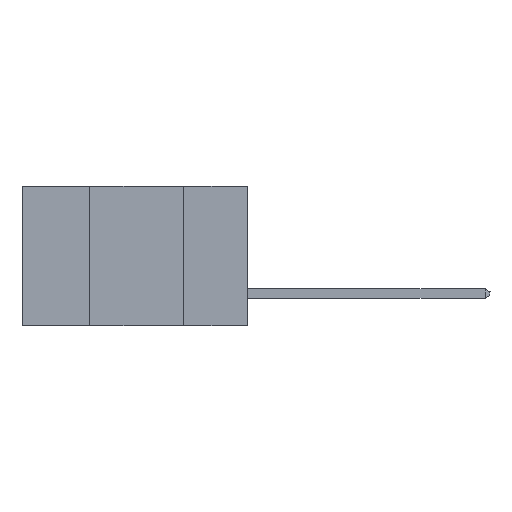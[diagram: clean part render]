
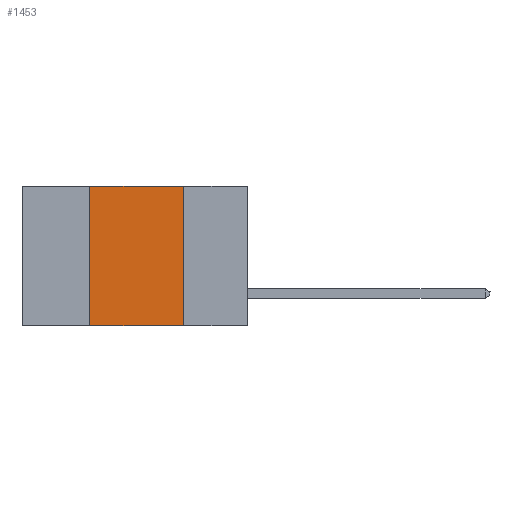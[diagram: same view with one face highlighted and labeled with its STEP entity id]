
A CAD part, left-side view. The second image highlights one B-rep face of the part: STEP entity #1453.
In plain terms, the highlighted planar face has unit normal (-1, 0, 0).
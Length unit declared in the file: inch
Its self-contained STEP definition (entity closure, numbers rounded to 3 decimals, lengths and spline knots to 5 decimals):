
#196 = DIRECTION ( 'NONE',  ( 0., -1., 0. ) ) ;
#423 = LINE ( 'NONE', #4731, #7227 ) ;
#1056 = VECTOR ( 'NONE', #19698, 39.37008 ) ;
#1349 = VERTEX_POINT ( 'NONE', #10973 ) ;
#1453 = ADVANCED_FACE ( 'NONE', ( #17598 ), #8153, .F. ) ;
#1739 = DIRECTION ( 'NONE',  ( 0., -1., 0. ) ) ;
#3515 = DIRECTION ( 'NONE',  ( 0., 0., -1. ) ) ;
#4006 = VERTEX_POINT ( 'NONE', #19813 ) ;
#4731 = CARTESIAN_POINT ( 'NONE',  ( 0., 0.17, -0.37 ) ) ;
#5026 = CARTESIAN_POINT ( 'NONE',  ( 0., 0.6, 0. ) ) ;
#5100 = LINE ( 'NONE', #5406, #1056 ) ;
#5406 = CARTESIAN_POINT ( 'NONE',  ( 0., 0.42, -0.37 ) ) ;
#6451 = CARTESIAN_POINT ( 'NONE',  ( 0., 0.6, 0. ) ) ;
#7102 = CARTESIAN_POINT ( 'NONE',  ( 0., 0.17, -0.37 ) ) ;
#7209 = EDGE_LOOP ( 'NONE', ( #10564, #15034, #8240, #12694 ) ) ;
#7227 = VECTOR ( 'NONE', #11128, 39.37008 ) ;
#7438 = VECTOR ( 'NONE', #196, 39.37008 ) ;
#8153 = PLANE ( 'NONE',  #9838 ) ;
#8240 = ORIENTED_EDGE ( 'NONE', *, *, #19629, .F. ) ;
#8712 = LINE ( 'NONE', #5026, #7438 ) ;
#9267 = EDGE_CURVE ( 'NONE', #4006, #17604, #423, .T. ) ;
#9838 = AXIS2_PLACEMENT_3D ( 'NONE', #6451, #9941, #3515 ) ;
#9941 = DIRECTION ( 'NONE',  ( 1., 0., 0. ) ) ;
#10063 = LINE ( 'NONE', #10166, #12621 ) ;
#10166 = CARTESIAN_POINT ( 'NONE',  ( 0., 0.6, -0.37 ) ) ;
#10564 = ORIENTED_EDGE ( 'NONE', *, *, #9267, .F. ) ;
#10910 = EDGE_CURVE ( 'NONE', #1349, #17604, #10063, .T. ) ;
#10973 = CARTESIAN_POINT ( 'NONE',  ( 0., 0.42, -0.37 ) ) ;
#11043 = VERTEX_POINT ( 'NONE', #13222 ) ;
#11128 = DIRECTION ( 'NONE',  ( 0., 0., -1. ) ) ;
#12621 = VECTOR ( 'NONE', #1739, 39.37008 ) ;
#12694 = ORIENTED_EDGE ( 'NONE', *, *, #10910, .T. ) ;
#13222 = CARTESIAN_POINT ( 'NONE',  ( 0., 0.42, 0. ) ) ;
#15034 = ORIENTED_EDGE ( 'NONE', *, *, #17180, .F. ) ;
#17180 = EDGE_CURVE ( 'NONE', #11043, #4006, #8712, .T. ) ;
#17598 = FACE_OUTER_BOUND ( 'NONE', #7209, .T. ) ;
#17604 = VERTEX_POINT ( 'NONE', #7102 ) ;
#19629 = EDGE_CURVE ( 'NONE', #1349, #11043, #5100, .T. ) ;
#19698 = DIRECTION ( 'NONE',  ( 0., 0., 1. ) ) ;
#19813 = CARTESIAN_POINT ( 'NONE',  ( 0., 0.17, 0. ) ) ;
